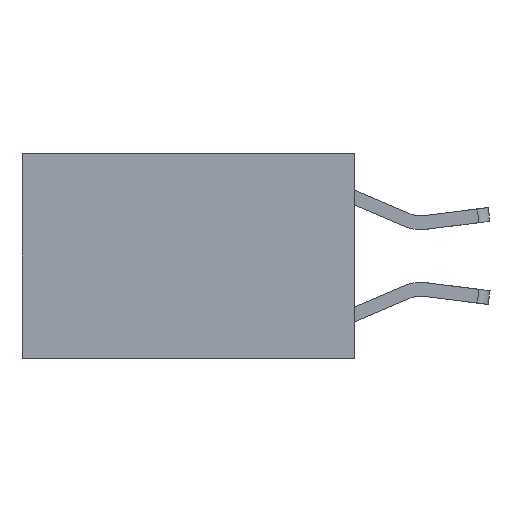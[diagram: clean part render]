
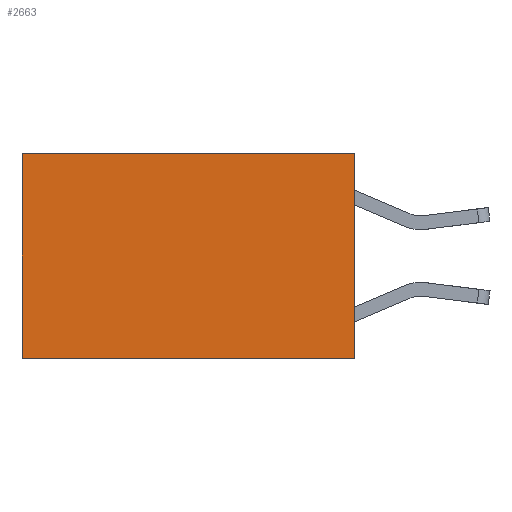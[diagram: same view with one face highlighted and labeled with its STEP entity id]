
A CAD part, left-side view. The second image highlights one B-rep face of the part: STEP entity #2663.
In plain terms, the highlighted planar face has unit normal (-1, 0, 0).
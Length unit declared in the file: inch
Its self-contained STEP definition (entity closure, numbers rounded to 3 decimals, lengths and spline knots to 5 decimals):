
#208 = ORIENTED_EDGE ( 'NONE', *, *, #3307, .F. ) ;
#1113 = VERTEX_POINT ( 'NONE', #4006 ) ;
#1552 = DIRECTION ( 'NONE',  ( 0., 0., -1. ) ) ;
#2171 = VECTOR ( 'NONE', #1552, 39.37008 ) ;
#2182 = VECTOR ( 'NONE', #12420, 39.37008 ) ;
#2663 = ADVANCED_FACE ( 'NONE', ( #4485 ), #6555, .F. ) ;
#2973 = DIRECTION ( 'NONE',  ( 1., 0., 0. ) ) ;
#3307 = EDGE_CURVE ( 'NONE', #10593, #4350, #6246, .T. ) ;
#3425 = VECTOR ( 'NONE', #5253, 39.37008 ) ;
#3781 = AXIS2_PLACEMENT_3D ( 'NONE', #12098, #2973, #8275 ) ;
#4006 = CARTESIAN_POINT ( 'NONE',  ( 0.2625, 0.6, -0.37 ) ) ;
#4350 = VERTEX_POINT ( 'NONE', #4760 ) ;
#4485 = FACE_OUTER_BOUND ( 'NONE', #6091, .T. ) ;
#4760 = CARTESIAN_POINT ( 'NONE',  ( 0.2625, 0., -0.37 ) ) ;
#5253 = DIRECTION ( 'NONE',  ( 0., 0., -1. ) ) ;
#5786 = CARTESIAN_POINT ( 'NONE',  ( 0.2625, 0., -0.37 ) ) ;
#6091 = EDGE_LOOP ( 'NONE', ( #12119, #9876, #208, #8356 ) ) ;
#6246 = LINE ( 'NONE', #8636, #3425 ) ;
#6555 = PLANE ( 'NONE',  #3781 ) ;
#7163 = EDGE_CURVE ( 'NONE', #10593, #10984, #12216, .T. ) ;
#7995 = EDGE_CURVE ( 'NONE', #4350, #1113, #9495, .T. ) ;
#8156 = CARTESIAN_POINT ( 'NONE',  ( 0.2625, 0., 0. ) ) ;
#8275 = DIRECTION ( 'NONE',  ( 0., 0., -1. ) ) ;
#8356 = ORIENTED_EDGE ( 'NONE', *, *, #7163, .T. ) ;
#8405 = CARTESIAN_POINT ( 'NONE',  ( 0.2625, 0., 0. ) ) ;
#8515 = EDGE_CURVE ( 'NONE', #10984, #1113, #12321, .T. ) ;
#8636 = CARTESIAN_POINT ( 'NONE',  ( 0.2625, 0., 0. ) ) ;
#9111 = DIRECTION ( 'NONE',  ( 0., 1., 0. ) ) ;
#9495 = LINE ( 'NONE', #5786, #2182 ) ;
#9671 = VECTOR ( 'NONE', #9111, 39.37008 ) ;
#9864 = CARTESIAN_POINT ( 'NONE',  ( 0.2625, 0.6, 0. ) ) ;
#9876 = ORIENTED_EDGE ( 'NONE', *, *, #7995, .F. ) ;
#10593 = VERTEX_POINT ( 'NONE', #8405 ) ;
#10984 = VERTEX_POINT ( 'NONE', #9864 ) ;
#11098 = CARTESIAN_POINT ( 'NONE',  ( 0.2625, 0.6, 0. ) ) ;
#12098 = CARTESIAN_POINT ( 'NONE',  ( 0.2625, 0., 0. ) ) ;
#12119 = ORIENTED_EDGE ( 'NONE', *, *, #8515, .T. ) ;
#12216 = LINE ( 'NONE', #8156, #9671 ) ;
#12321 = LINE ( 'NONE', #11098, #2171 ) ;
#12420 = DIRECTION ( 'NONE',  ( 0., 1., 0. ) ) ;
